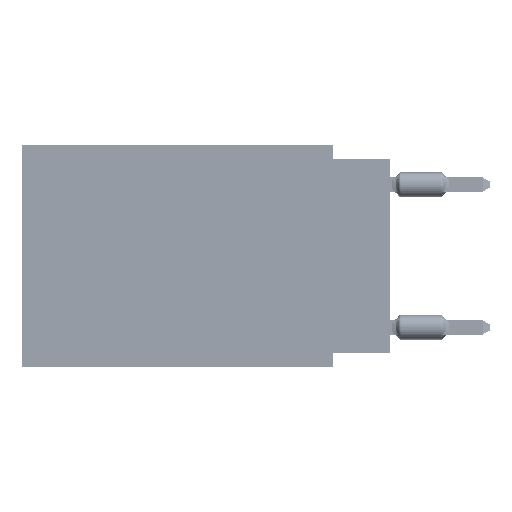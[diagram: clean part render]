
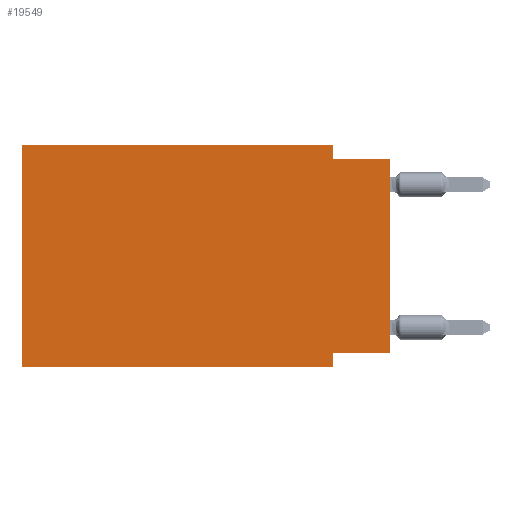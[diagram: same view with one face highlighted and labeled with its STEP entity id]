
A CAD part, left-side view. The second image highlights one B-rep face of the part: STEP entity #19549.
In plain terms, the highlighted planar face has unit normal (-1, 0, 0).
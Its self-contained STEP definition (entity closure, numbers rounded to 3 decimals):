
#144 = VERTEX_POINT ( 'NONE', #48004 ) ;
#995 = DIRECTION ( 'NONE',  ( 0., -1., 0. ) ) ;
#1366 = DIRECTION ( 'NONE',  ( 0., 0., -1. ) ) ;
#1832 = EDGE_CURVE ( 'NONE', #64011, #144, #13964, .T. ) ;
#2147 = LINE ( 'NONE', #19514, #65609 ) ;
#6149 = CARTESIAN_POINT ( 'NONE',  ( 0., 2.54, -9.906 ) ) ;
#6847 = EDGE_CURVE ( 'NONE', #64011, #34357, #71970, .T. ) ;
#7724 = CARTESIAN_POINT ( 'NONE',  ( 0., 16.383, -9.906 ) ) ;
#7820 = ORIENTED_EDGE ( 'NONE', *, *, #72715, .F. ) ;
#9643 = VECTOR ( 'NONE', #22269, 1000. ) ;
#11806 = DIRECTION ( 'NONE',  ( 0., 0., 1. ) ) ;
#13655 = EDGE_CURVE ( 'NONE', #29263, #56619, #2147, .T. ) ;
#13964 = LINE ( 'NONE', #40527, #32997 ) ;
#15245 = LINE ( 'NONE', #38276, #71991 ) ;
#17556 = EDGE_CURVE ( 'NONE', #54629, #74203, #45431, .T. ) ;
#19107 = CARTESIAN_POINT ( 'NONE',  ( 0., 16.383, 0. ) ) ;
#19514 = CARTESIAN_POINT ( 'NONE',  ( 0., 2.54, 0. ) ) ;
#19549 = ADVANCED_FACE ( 'NONE', ( #53846 ), #58758, .F. ) ;
#20113 = LINE ( 'NONE', #60887, #29805 ) ;
#20479 = DIRECTION ( 'NONE',  ( 0., -1., 0. ) ) ;
#20780 = VERTEX_POINT ( 'NONE', #59520 ) ;
#22269 = DIRECTION ( 'NONE',  ( 0., 0., 1. ) ) ;
#23676 = LINE ( 'NONE', #19107, #45073 ) ;
#25512 = EDGE_CURVE ( 'NONE', #20780, #29263, #23676, .T. ) ;
#28256 = EDGE_CURVE ( 'NONE', #56619, #144, #20113, .T. ) ;
#29263 = VERTEX_POINT ( 'NONE', #64325 ) ;
#29805 = VECTOR ( 'NONE', #20479, 1000. ) ;
#30056 = EDGE_CURVE ( 'NONE', #54629, #20780, #33239, .T. ) ;
#30217 = AXIS2_PLACEMENT_3D ( 'NONE', #42516, #53083, #1366 ) ;
#31189 = VECTOR ( 'NONE', #48013, 1000. ) ;
#32997 = VECTOR ( 'NONE', #11806, 1000. ) ;
#33239 = LINE ( 'NONE', #33602, #9643 ) ;
#33602 = CARTESIAN_POINT ( 'NONE',  ( 0., 16.383, 0. ) ) ;
#33776 = ORIENTED_EDGE ( 'NONE', *, *, #17556, .T. ) ;
#34357 = VERTEX_POINT ( 'NONE', #54885 ) ;
#35424 = DIRECTION ( 'NONE',  ( 0., 0., -1. ) ) ;
#36511 = DIRECTION ( 'NONE',  ( 0., 1., 0. ) ) ;
#37352 = ORIENTED_EDGE ( 'NONE', *, *, #1832, .T. ) ;
#38276 = CARTESIAN_POINT ( 'NONE',  ( 0., 2.54, -9.906 ) ) ;
#39033 = ORIENTED_EDGE ( 'NONE', *, *, #6847, .F. ) ;
#40525 = CARTESIAN_POINT ( 'NONE',  ( 0., 16.383, -9.906 ) ) ;
#40527 = CARTESIAN_POINT ( 'NONE',  ( 0., 0., 0. ) ) ;
#42152 = CARTESIAN_POINT ( 'NONE',  ( 0., 0., -9.271 ) ) ;
#42516 = CARTESIAN_POINT ( 'NONE',  ( 0., 16.383, 0. ) ) ;
#44188 = VECTOR ( 'NONE', #36511, 1000. ) ;
#45073 = VECTOR ( 'NONE', #995, 1000. ) ;
#45344 = EDGE_LOOP ( 'NONE', ( #37352, #74220, #52274, #65161, #70585, #33776, #7820, #39033 ) ) ;
#45431 = LINE ( 'NONE', #40525, #31189 ) ;
#48004 = CARTESIAN_POINT ( 'NONE',  ( 0., 0., -0.635 ) ) ;
#48013 = DIRECTION ( 'NONE',  ( 0., -1., 0. ) ) ;
#52274 = ORIENTED_EDGE ( 'NONE', *, *, #13655, .F. ) ;
#53083 = DIRECTION ( 'NONE',  ( 1., 0., 0. ) ) ;
#53846 = FACE_OUTER_BOUND ( 'NONE', #45344, .T. ) ;
#54629 = VERTEX_POINT ( 'NONE', #7724 ) ;
#54885 = CARTESIAN_POINT ( 'NONE',  ( 0., 2.54, -9.271 ) ) ;
#56619 = VERTEX_POINT ( 'NONE', #67895 ) ;
#58758 = PLANE ( 'NONE',  #30217 ) ;
#59520 = CARTESIAN_POINT ( 'NONE',  ( 0., 16.383, 0. ) ) ;
#60887 = CARTESIAN_POINT ( 'NONE',  ( 0., 0., -0.635 ) ) ;
#61304 = DIRECTION ( 'NONE',  ( 0., 0., -1. ) ) ;
#64011 = VERTEX_POINT ( 'NONE', #72461 ) ;
#64325 = CARTESIAN_POINT ( 'NONE',  ( 0., 2.54, 0. ) ) ;
#65161 = ORIENTED_EDGE ( 'NONE', *, *, #25512, .F. ) ;
#65609 = VECTOR ( 'NONE', #35424, 1000. ) ;
#67895 = CARTESIAN_POINT ( 'NONE',  ( 0., 2.54, -0.635 ) ) ;
#70585 = ORIENTED_EDGE ( 'NONE', *, *, #30056, .F. ) ;
#71970 = LINE ( 'NONE', #42152, #44188 ) ;
#71991 = VECTOR ( 'NONE', #61304, 1000. ) ;
#72461 = CARTESIAN_POINT ( 'NONE',  ( 0., 0., -9.271 ) ) ;
#72715 = EDGE_CURVE ( 'NONE', #34357, #74203, #15245, .T. ) ;
#74203 = VERTEX_POINT ( 'NONE', #6149 ) ;
#74220 = ORIENTED_EDGE ( 'NONE', *, *, #28256, .F. ) ;
